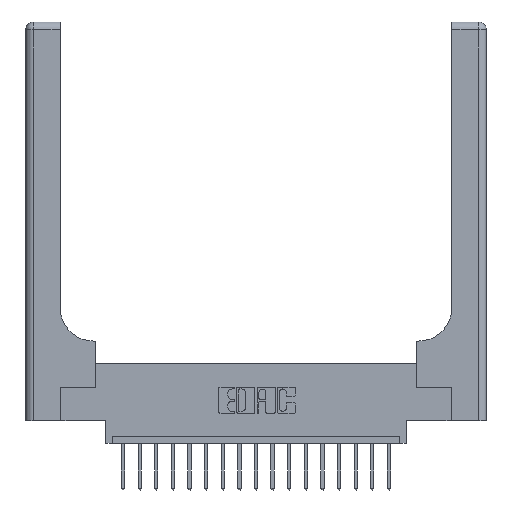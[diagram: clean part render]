
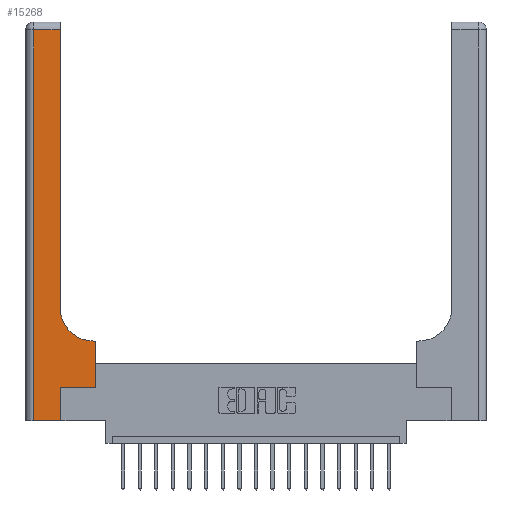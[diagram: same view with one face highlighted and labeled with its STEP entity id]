
A CAD part, top view. The second image highlights one B-rep face of the part: STEP entity #15268.
In plain terms, the highlighted planar face has unit normal (0, 0, 1).
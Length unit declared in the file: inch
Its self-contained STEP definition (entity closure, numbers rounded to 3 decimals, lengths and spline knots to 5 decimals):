
#86 = FACE_OUTER_BOUND ( 'NONE', #12851, .T. ) ;
#126 = LINE ( 'NONE', #5003, #13600 ) ;
#181 = CARTESIAN_POINT ( 'NONE',  ( 0.265, 0., 0.37 ) ) ;
#233 = CARTESIAN_POINT ( 'NONE',  ( 0.265, 0.25, 0.37 ) ) ;
#428 = DIRECTION ( 'NONE',  ( 1., 0., 0. ) ) ;
#782 = VERTEX_POINT ( 'NONE', #16117 ) ;
#1268 = EDGE_CURVE ( 'NONE', #782, #16177, #14172, .T. ) ;
#1751 = VECTOR ( 'NONE', #5648, 39.37008 ) ;
#1942 = CARTESIAN_POINT ( 'NONE',  ( 0.26, 2.94, 0.37 ) ) ;
#1965 = EDGE_CURVE ( 'NONE', #6204, #5493, #6136, .T. ) ;
#2015 = CARTESIAN_POINT ( 'NONE',  ( 0.528, 0.25, 0.37 ) ) ;
#2570 = ORIENTED_EDGE ( 'NONE', *, *, #5498, .T. ) ;
#3210 = LINE ( 'NONE', #233, #19540 ) ;
#3603 = DIRECTION ( 'NONE',  ( -1., 0., 0. ) ) ;
#3815 = VERTEX_POINT ( 'NONE', #2015 ) ;
#3896 = CARTESIAN_POINT ( 'NONE',  ( 0.51, 0.6, 0.37 ) ) ;
#3948 = LINE ( 'NONE', #11425, #12481 ) ;
#4140 = VECTOR ( 'NONE', #3603, 39.37008 ) ;
#4189 = CARTESIAN_POINT ( 'NONE',  ( 0.06, 2.94, 0.37 ) ) ;
#4562 = PLANE ( 'NONE',  #11784 ) ;
#4734 = CARTESIAN_POINT ( 'NONE',  ( 0.265, 0., 0.37 ) ) ;
#4970 = CARTESIAN_POINT ( 'NONE',  ( 0.51, 0.85, 0.37 ) ) ;
#5003 = CARTESIAN_POINT ( 'NONE',  ( 0., 0., 0.37 ) ) ;
#5169 = DIRECTION ( 'NONE',  ( 0., 1., 0. ) ) ;
#5493 = VERTEX_POINT ( 'NONE', #17534 ) ;
#5498 = EDGE_CURVE ( 'NONE', #12354, #8797, #10366, .T. ) ;
#5648 = DIRECTION ( 'NONE',  ( 0., 1., 0. ) ) ;
#5774 = DIRECTION ( 'NONE',  ( 0., -1., 0. ) ) ;
#6136 = LINE ( 'NONE', #181, #16661 ) ;
#6204 = VERTEX_POINT ( 'NONE', #4734 ) ;
#6223 = ORIENTED_EDGE ( 'NONE', *, *, #13403, .T. ) ;
#6240 = DIRECTION ( 'NONE',  ( 0., 1., 0. ) ) ;
#6660 = DIRECTION ( 'NONE',  ( 1., 0., 0. ) ) ;
#7611 = CARTESIAN_POINT ( 'NONE',  ( 0.26, 0.6, 0.37 ) ) ;
#7941 = DIRECTION ( 'NONE',  ( -1., 0., 0. ) ) ;
#7994 = ORIENTED_EDGE ( 'NONE', *, *, #9505, .T. ) ;
#8688 = ORIENTED_EDGE ( 'NONE', *, *, #16950, .T. ) ;
#8725 = LINE ( 'NONE', #13412, #1751 ) ;
#8780 = VERTEX_POINT ( 'NONE', #17493 ) ;
#8797 = VERTEX_POINT ( 'NONE', #18998 ) ;
#9283 = VECTOR ( 'NONE', #5774, 39.37008 ) ;
#9493 = DIRECTION ( 'NONE',  ( 1., 0., 0. ) ) ;
#9505 = EDGE_CURVE ( 'NONE', #3815, #782, #17326, .T. ) ;
#10030 = DIRECTION ( 'NONE',  ( -1., 0., 0. ) ) ;
#10366 = LINE ( 'NONE', #17828, #9283 ) ;
#10884 = ORIENTED_EDGE ( 'NONE', *, *, #11132, .T. ) ;
#11132 = EDGE_CURVE ( 'NONE', #8780, #15857, #8725, .T. ) ;
#11359 = CARTESIAN_POINT ( 'NONE',  ( 0.528, 0.25, 0.37 ) ) ;
#11425 = CARTESIAN_POINT ( 'NONE',  ( 0., 2.94, 0.37 ) ) ;
#11784 = AXIS2_PLACEMENT_3D ( 'NONE', #18314, #16915, #7941 ) ;
#12354 = VERTEX_POINT ( 'NONE', #4189 ) ;
#12481 = VECTOR ( 'NONE', #10030, 39.37008 ) ;
#12851 = EDGE_LOOP ( 'NONE', ( #10884, #19421, #2570, #6223, #13709, #19333, #7994, #15350, #8688 ) ) ;
#13403 = EDGE_CURVE ( 'NONE', #8797, #6204, #126, .T. ) ;
#13412 = CARTESIAN_POINT ( 'NONE',  ( 0.26, 3., 0.37 ) ) ;
#13600 = VECTOR ( 'NONE', #428, 39.37008 ) ;
#13709 = ORIENTED_EDGE ( 'NONE', *, *, #1965, .T. ) ;
#13942 = DIRECTION ( 'NONE',  ( 0., 0., -1. ) ) ;
#14108 = AXIS2_PLACEMENT_3D ( 'NONE', #4970, #13942, #6660 ) ;
#14172 = LINE ( 'NONE', #7611, #4140 ) ;
#14489 = VECTOR ( 'NONE', #5169, 39.37008 ) ;
#15268 = ADVANCED_FACE ( 'NONE', ( #86 ), #4562, .F. ) ;
#15350 = ORIENTED_EDGE ( 'NONE', *, *, #1268, .T. ) ;
#15857 = VERTEX_POINT ( 'NONE', #1942 ) ;
#16117 = CARTESIAN_POINT ( 'NONE',  ( 0.528, 0.6, 0.37 ) ) ;
#16177 = VERTEX_POINT ( 'NONE', #3896 ) ;
#16225 = EDGE_CURVE ( 'NONE', #15857, #12354, #3948, .T. ) ;
#16661 = VECTOR ( 'NONE', #6240, 39.37008 ) ;
#16915 = DIRECTION ( 'NONE',  ( 0., 0., -1. ) ) ;
#16950 = EDGE_CURVE ( 'NONE', #16177, #8780, #17921, .T. ) ;
#17326 = LINE ( 'NONE', #11359, #14489 ) ;
#17493 = CARTESIAN_POINT ( 'NONE',  ( 0.26, 0.85, 0.37 ) ) ;
#17534 = CARTESIAN_POINT ( 'NONE',  ( 0.265, 0.25, 0.37 ) ) ;
#17828 = CARTESIAN_POINT ( 'NONE',  ( 0.06, 3., 0.37 ) ) ;
#17921 = CIRCLE ( 'NONE', #14108, 0.25 ) ;
#18314 = CARTESIAN_POINT ( 'NONE',  ( 0., 3., 0.37 ) ) ;
#18998 = CARTESIAN_POINT ( 'NONE',  ( 0.06, 0., 0.37 ) ) ;
#19333 = ORIENTED_EDGE ( 'NONE', *, *, #19453, .T. ) ;
#19421 = ORIENTED_EDGE ( 'NONE', *, *, #16225, .T. ) ;
#19453 = EDGE_CURVE ( 'NONE', #5493, #3815, #3210, .T. ) ;
#19540 = VECTOR ( 'NONE', #9493, 39.37008 ) ;
